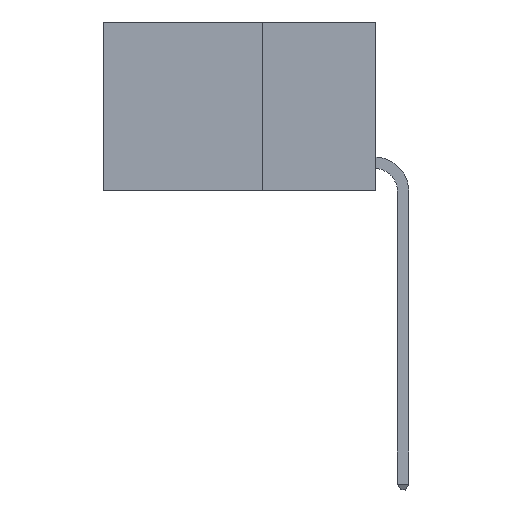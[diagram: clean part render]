
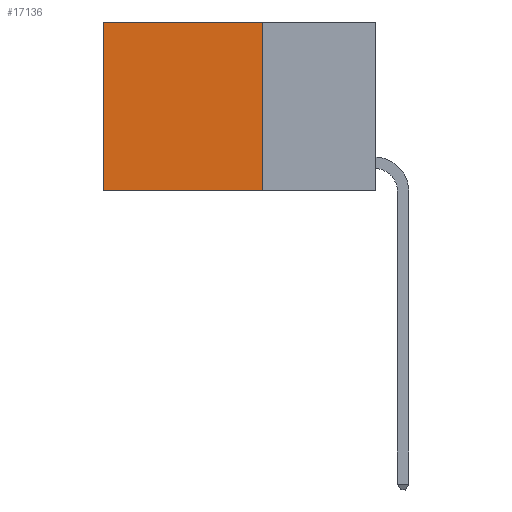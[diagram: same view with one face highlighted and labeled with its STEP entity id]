
A CAD part, left-side view. The second image highlights one B-rep face of the part: STEP entity #17136.
In plain terms, the highlighted planar face has unit normal (-1, 0, 0).
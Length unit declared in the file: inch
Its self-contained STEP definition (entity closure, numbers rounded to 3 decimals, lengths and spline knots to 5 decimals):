
#186 = DIRECTION ( 'NONE',  ( 0., 0., -1. ) ) ;
#827 = VERTEX_POINT ( 'NONE', #9885 ) ;
#1561 = EDGE_CURVE ( 'NONE', #5990, #7255, #11806, .T. ) ;
#1687 = VERTEX_POINT ( 'NONE', #14480 ) ;
#2353 = DIRECTION ( 'NONE',  ( 1., 0., 0. ) ) ;
#3523 = EDGE_CURVE ( 'NONE', #1687, #5990, #4936, .T. ) ;
#4242 = EDGE_CURVE ( 'NONE', #1687, #827, #9722, .T. ) ;
#4311 = AXIS2_PLACEMENT_3D ( 'NONE', #5499, #2353, #17699 ) ;
#4442 = VECTOR ( 'NONE', #8517, 39.37008 ) ;
#4936 = LINE ( 'NONE', #8953, #4442 ) ;
#5499 = CARTESIAN_POINT ( 'NONE',  ( 0.2625, 0.25, 0. ) ) ;
#5990 = VERTEX_POINT ( 'NONE', #15674 ) ;
#6784 = CARTESIAN_POINT ( 'NONE',  ( 0.2625, 0.6, 0. ) ) ;
#7068 = PLANE ( 'NONE',  #4311 ) ;
#7213 = VECTOR ( 'NONE', #186, 39.37008 ) ;
#7255 = VERTEX_POINT ( 'NONE', #18485 ) ;
#7768 = CARTESIAN_POINT ( 'NONE',  ( 0.2625, 0.25, -0.37 ) ) ;
#7829 = DIRECTION ( 'NONE',  ( 0., 1., 0. ) ) ;
#8308 = DIRECTION ( 'NONE',  ( 0., 0., -1. ) ) ;
#8517 = DIRECTION ( 'NONE',  ( 0., 1., 0. ) ) ;
#8953 = CARTESIAN_POINT ( 'NONE',  ( 0.2625, 0.25, 0. ) ) ;
#9722 = LINE ( 'NONE', #9861, #17289 ) ;
#9861 = CARTESIAN_POINT ( 'NONE',  ( 0.2625, 0.25, 0. ) ) ;
#9885 = CARTESIAN_POINT ( 'NONE',  ( 0.2625, 0.25, -0.37 ) ) ;
#11052 = EDGE_CURVE ( 'NONE', #827, #7255, #16929, .T. ) ;
#11806 = LINE ( 'NONE', #6784, #7213 ) ;
#12917 = VECTOR ( 'NONE', #7829, 39.37008 ) ;
#14480 = CARTESIAN_POINT ( 'NONE',  ( 0.2625, 0.25, 0. ) ) ;
#15674 = CARTESIAN_POINT ( 'NONE',  ( 0.2625, 0.6, 0. ) ) ;
#15858 = EDGE_LOOP ( 'NONE', ( #16065, #18970, #17040, #16382 ) ) ;
#16065 = ORIENTED_EDGE ( 'NONE', *, *, #1561, .T. ) ;
#16382 = ORIENTED_EDGE ( 'NONE', *, *, #3523, .T. ) ;
#16929 = LINE ( 'NONE', #7768, #12917 ) ;
#17040 = ORIENTED_EDGE ( 'NONE', *, *, #4242, .F. ) ;
#17136 = ADVANCED_FACE ( 'NONE', ( #17347 ), #7068, .F. ) ;
#17289 = VECTOR ( 'NONE', #8308, 39.37008 ) ;
#17347 = FACE_OUTER_BOUND ( 'NONE', #15858, .T. ) ;
#17699 = DIRECTION ( 'NONE',  ( 0., 0., -1. ) ) ;
#18485 = CARTESIAN_POINT ( 'NONE',  ( 0.2625, 0.6, -0.37 ) ) ;
#18970 = ORIENTED_EDGE ( 'NONE', *, *, #11052, .F. ) ;
